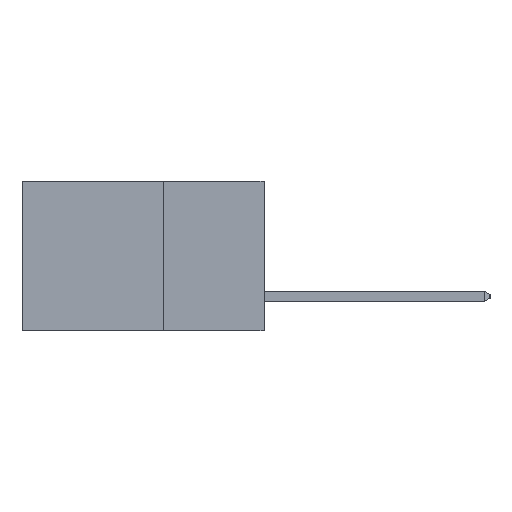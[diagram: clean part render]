
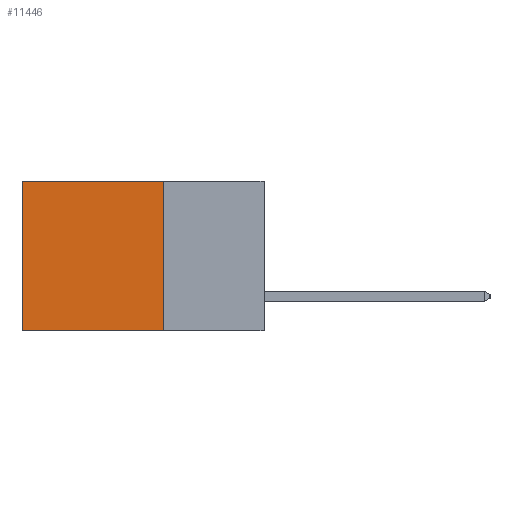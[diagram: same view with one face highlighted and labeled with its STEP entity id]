
A CAD part, left-side view. The second image highlights one B-rep face of the part: STEP entity #11446.
In plain terms, the highlighted planar face has unit normal (-1, 0, 0).
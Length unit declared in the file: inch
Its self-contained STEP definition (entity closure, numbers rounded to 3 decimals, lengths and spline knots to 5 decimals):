
#271 = FACE_OUTER_BOUND ( 'NONE', #19581, .T. ) ;
#293 = CARTESIAN_POINT ( 'NONE',  ( 0.2615, 0.6, 0. ) ) ;
#308 = DIRECTION ( 'NONE',  ( 0., 1., 0. ) ) ;
#1994 = ORIENTED_EDGE ( 'NONE', *, *, #8133, .F. ) ;
#2852 = VECTOR ( 'NONE', #15736, 39.37008 ) ;
#3385 = LINE ( 'NONE', #15363, #2852 ) ;
#4247 = ORIENTED_EDGE ( 'NONE', *, *, #11340, .F. ) ;
#5768 = LINE ( 'NONE', #10303, #14010 ) ;
#7238 = CARTESIAN_POINT ( 'NONE',  ( 0.2615, 0.25, 0. ) ) ;
#8133 = EDGE_CURVE ( 'NONE', #20140, #15862, #3385, .T. ) ;
#8281 = LINE ( 'NONE', #15812, #12443 ) ;
#9834 = EDGE_CURVE ( 'NONE', #13791, #12520, #5768, .T. ) ;
#10303 = CARTESIAN_POINT ( 'NONE',  ( 0.2615, 0.6, -0.37 ) ) ;
#11340 = EDGE_CURVE ( 'NONE', #15862, #12520, #8281, .T. ) ;
#11446 = ADVANCED_FACE ( 'NONE', ( #271 ), #20395, .F. ) ;
#11655 = CARTESIAN_POINT ( 'NONE',  ( 0.2615, 0.6, -0.37 ) ) ;
#11707 = DIRECTION ( 'NONE',  ( 0., 0., -1. ) ) ;
#12443 = VECTOR ( 'NONE', #19292, 39.37008 ) ;
#12520 = VERTEX_POINT ( 'NONE', #11655 ) ;
#12678 = AXIS2_PLACEMENT_3D ( 'NONE', #20374, #20326, #20319 ) ;
#13359 = ORIENTED_EDGE ( 'NONE', *, *, #9834, .T. ) ;
#13506 = CARTESIAN_POINT ( 'NONE',  ( 0.2615, 0.25, -0.37 ) ) ;
#13791 = VERTEX_POINT ( 'NONE', #293 ) ;
#14010 = VECTOR ( 'NONE', #11707, 39.37008 ) ;
#15363 = CARTESIAN_POINT ( 'NONE',  ( 0.2615, 0.25, -0.37 ) ) ;
#15398 = LINE ( 'NONE', #21103, #18818 ) ;
#15736 = DIRECTION ( 'NONE',  ( 0., 0., -1. ) ) ;
#15812 = CARTESIAN_POINT ( 'NONE',  ( 0.2615, 0.25, -0.37 ) ) ;
#15862 = VERTEX_POINT ( 'NONE', #13506 ) ;
#18818 = VECTOR ( 'NONE', #308, 39.37008 ) ;
#19264 = EDGE_CURVE ( 'NONE', #20140, #13791, #15398, .T. ) ;
#19292 = DIRECTION ( 'NONE',  ( 0., 1., 0. ) ) ;
#19581 = EDGE_LOOP ( 'NONE', ( #13359, #4247, #1994, #21044 ) ) ;
#20140 = VERTEX_POINT ( 'NONE', #7238 ) ;
#20319 = DIRECTION ( 'NONE',  ( 0., 0., -1. ) ) ;
#20326 = DIRECTION ( 'NONE',  ( 1., 0., 0. ) ) ;
#20374 = CARTESIAN_POINT ( 'NONE',  ( 0.2615, 0.25, -0.37 ) ) ;
#20395 = PLANE ( 'NONE',  #12678 ) ;
#21044 = ORIENTED_EDGE ( 'NONE', *, *, #19264, .T. ) ;
#21103 = CARTESIAN_POINT ( 'NONE',  ( 0.2615, 0.25, 0. ) ) ;
